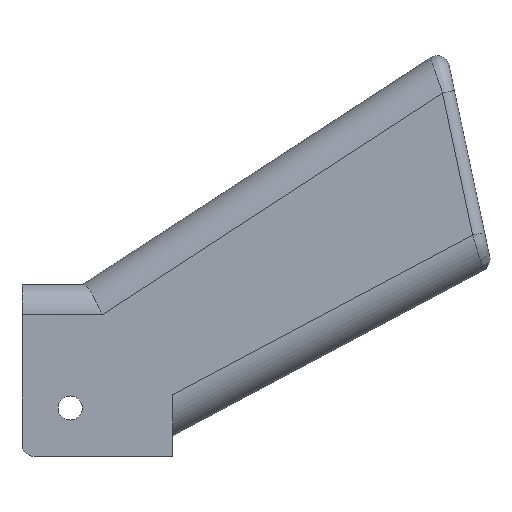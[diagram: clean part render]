
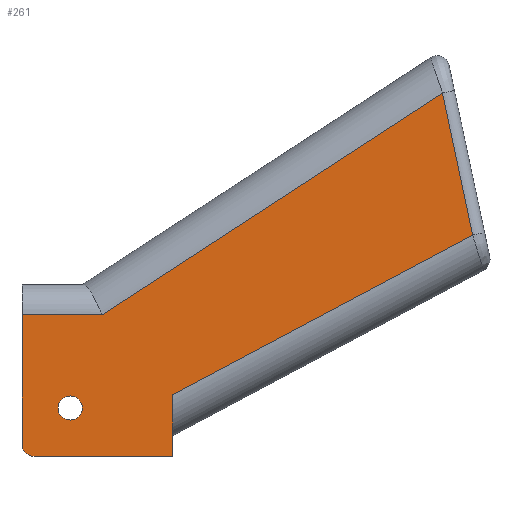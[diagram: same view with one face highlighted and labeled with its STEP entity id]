
A CAD part, left-side view. The second image highlights one B-rep face of the part: STEP entity #261.
In plain terms, the highlighted planar face has unit normal (-1, 0, 0).
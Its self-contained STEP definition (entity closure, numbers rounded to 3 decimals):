
#108 = CARTESIAN_POINT ( 'NONE',  ( -11.112, 29.21, -16.51 ) ) ;
#111 = VECTOR ( 'NONE', #488, 1000. ) ;
#127 = DIRECTION ( 'NONE',  ( 1., 0., 0. ) ) ;
#141 = LINE ( 'NONE', #618, #111 ) ;
#261 = ADVANCED_FACE ( 'NONE', ( #1102, #1049 ), #744, .F. ) ;
#338 = CARTESIAN_POINT ( 'NONE',  ( -11.112, 21.59, -6.35 ) ) ;
#363 = VERTEX_POINT ( 'NONE', #1512 ) ;
#379 = CARTESIAN_POINT ( 'NONE',  ( -11.112, 0., -16.51 ) ) ;
#403 = CARTESIAN_POINT ( 'NONE',  ( -11.112, 0., -3.562 ) ) ;
#422 = CARTESIAN_POINT ( 'NONE',  ( -11.112, 21.59, -3.81 ) ) ;
#456 = VECTOR ( 'NONE', #1524, 1000. ) ;
#475 = LINE ( 'NONE', #1577, #456 ) ;
#484 = DIRECTION ( 'NONE',  ( 0., 0., 1. ) ) ;
#488 = DIRECTION ( 'NONE',  ( 0., 0.838, -0.546 ) ) ;
#503 = CARTESIAN_POINT ( 'NONE',  ( -11.112, 21.59, -8.89 ) ) ;
#539 = AXIS2_PLACEMENT_3D ( 'NONE', #338, #1357, #484 ) ;
#608 = EDGE_LOOP ( 'NONE', ( #751, #753 ) ) ;
#618 = CARTESIAN_POINT ( 'NONE',  ( -11.112, 2.966, 21.065 ) ) ;
#627 = CARTESIAN_POINT ( 'NONE',  ( -11.112, 0., 16.51 ) ) ;
#656 = VERTEX_POINT ( 'NONE', #1812 ) ;
#671 = DIRECTION ( 'NONE',  ( 0., 0., -1. ) ) ;
#679 = DIRECTION ( 'NONE',  ( -1., 0., 0. ) ) ;
#689 = CARTESIAN_POINT ( 'NONE',  ( -11.112, 29.21, -13.97 ) ) ;
#706 = AXIS2_PLACEMENT_3D ( 'NONE', #689, #679, #671 ) ;
#715 = AXIS2_PLACEMENT_3D ( 'NONE', #1107, #1100, #1091 ) ;
#728 = EDGE_CURVE ( 'NONE', #1424, #1757, #1784, .T. ) ;
#733 = DIRECTION ( 'NONE',  ( 0., 0., -1. ) ) ;
#744 = PLANE ( 'NONE',  #1173 ) ;
#751 = ORIENTED_EDGE ( 'NONE', *, *, #1468, .F. ) ;
#753 = ORIENTED_EDGE ( 'NONE', *, *, #1752, .F. ) ;
#755 = ORIENTED_EDGE ( 'NONE', *, *, #728, .T. ) ;
#777 = ORIENTED_EDGE ( 'NONE', *, *, #1492, .T. ) ;
#779 = ORIENTED_EDGE ( 'NONE', *, *, #1449, .T. ) ;
#787 = CARTESIAN_POINT ( 'NONE',  ( -11.112, 0., 16.51 ) ) ;
#795 = CIRCLE ( 'NONE', #706, 2.54 ) ;
#797 = ORIENTED_EDGE ( 'NONE', *, *, #1759, .F. ) ;
#799 = ORIENTED_EDGE ( 'NONE', *, *, #1438, .T. ) ;
#826 = ORIENTED_EDGE ( 'NONE', *, *, #1462, .T. ) ;
#830 = ORIENTED_EDGE ( 'NONE', *, *, #1621, .T. ) ;
#854 = ORIENTED_EDGE ( 'NONE', *, *, #1555, .T. ) ;
#866 = VECTOR ( 'NONE', #1232, 1000. ) ;
#872 = VERTEX_POINT ( 'NONE', #1733 ) ;
#887 = CIRCLE ( 'NONE', #715, 2.54 ) ;
#906 = LINE ( 'NONE', #1358, #866 ) ;
#934 = VECTOR ( 'NONE', #1419, 1000. ) ;
#963 = VERTEX_POINT ( 'NONE', #422 ) ;
#993 = LINE ( 'NONE', #1437, #934 ) ;
#1016 = VECTOR ( 'NONE', #1557, 1000. ) ;
#1045 = LINE ( 'NONE', #627, #1798 ) ;
#1049 = FACE_OUTER_BOUND ( 'NONE', #1734, .T. ) ;
#1053 = VERTEX_POINT ( 'NONE', #503 ) ;
#1055 = LINE ( 'NONE', #1642, #1016 ) ;
#1064 = CIRCLE ( 'NONE', #539, 2.54 ) ;
#1072 = CARTESIAN_POINT ( 'NONE',  ( -11.112, 31.75, -13.97 ) ) ;
#1077 = VERTEX_POINT ( 'NONE', #403 ) ;
#1091 = DIRECTION ( 'NONE',  ( 0., 0., 1. ) ) ;
#1100 = DIRECTION ( 'NONE',  ( -1., 0., 0. ) ) ;
#1102 = FACE_BOUND ( 'NONE', #608, .T. ) ;
#1107 = CARTESIAN_POINT ( 'NONE',  ( -11.112, 21.59, -6.35 ) ) ;
#1173 = AXIS2_PLACEMENT_3D ( 'NONE', #787, #127, #733 ) ;
#1232 = DIRECTION ( 'NONE',  ( 0., 0.208, 0.978 ) ) ;
#1357 = DIRECTION ( 'NONE',  ( -1., 0., 0. ) ) ;
#1358 = CARTESIAN_POINT ( 'NONE',  ( -11.112, -63.326, 29.97 ) ) ;
#1381 = CARTESIAN_POINT ( 'NONE',  ( -11.112, 31.75, 16.51 ) ) ;
#1419 = DIRECTION ( 'NONE',  ( 0., -1., 0. ) ) ;
#1421 = VERTEX_POINT ( 'NONE', #108 ) ;
#1424 = VERTEX_POINT ( 'NONE', #1876 ) ;
#1429 = DIRECTION ( 'NONE',  ( 0., 0., -1. ) ) ;
#1437 = CARTESIAN_POINT ( 'NONE',  ( -11.112, 0., -16.51 ) ) ;
#1438 = EDGE_CURVE ( 'NONE', #1077, #363, #1055, .T. ) ;
#1449 = EDGE_CURVE ( 'NONE', #1421, #1891, #993, .T. ) ;
#1462 = EDGE_CURVE ( 'NONE', #363, #872, #906, .T. ) ;
#1468 = EDGE_CURVE ( 'NONE', #963, #1053, #887, .T. ) ;
#1492 = EDGE_CURVE ( 'NONE', #1757, #1421, #795, .T. ) ;
#1512 = CARTESIAN_POINT ( 'NONE',  ( -11.112, -63.299, 30.095 ) ) ;
#1524 = DIRECTION ( 'NONE',  ( 0., 1., 0. ) ) ;
#1555 = EDGE_CURVE ( 'NONE', #656, #1424, #475, .T. ) ;
#1557 = DIRECTION ( 'NONE',  ( 0., -0.883, 0.469 ) ) ;
#1577 = CARTESIAN_POINT ( 'NONE',  ( -11.112, 31.75, 13.335 ) ) ;
#1621 = EDGE_CURVE ( 'NONE', #872, #656, #141, .T. ) ;
#1642 = CARTESIAN_POINT ( 'NONE',  ( -11.112, -8.32, 0.862 ) ) ;
#1733 = CARTESIAN_POINT ( 'NONE',  ( -11.112, -56.929, 60.065 ) ) ;
#1734 = EDGE_LOOP ( 'NONE', ( #755, #777, #779, #797, #799, #826, #830, #854 ) ) ;
#1752 = EDGE_CURVE ( 'NONE', #1053, #963, #1064, .T. ) ;
#1757 = VERTEX_POINT ( 'NONE', #1072 ) ;
#1759 = EDGE_CURVE ( 'NONE', #1077, #1891, #1045, .T. ) ;
#1762 = VECTOR ( 'NONE', #1429, 1000. ) ;
#1784 = LINE ( 'NONE', #1381, #1762 ) ;
#1798 = VECTOR ( 'NONE', #1811, 1000. ) ;
#1811 = DIRECTION ( 'NONE',  ( 0., 0., -1. ) ) ;
#1812 = CARTESIAN_POINT ( 'NONE',  ( -11.112, 14.837, 13.335 ) ) ;
#1876 = CARTESIAN_POINT ( 'NONE',  ( -11.112, 31.75, 13.335 ) ) ;
#1891 = VERTEX_POINT ( 'NONE', #379 ) ;
